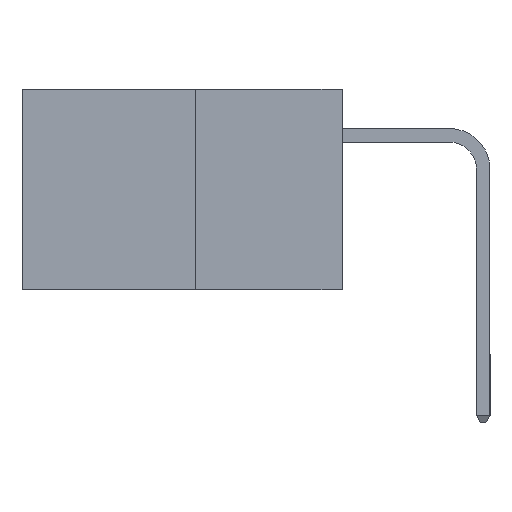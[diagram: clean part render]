
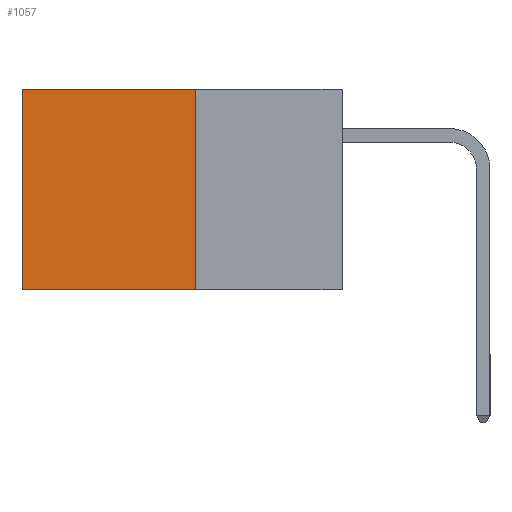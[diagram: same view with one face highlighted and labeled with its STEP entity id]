
A CAD part, left-side view. The second image highlights one B-rep face of the part: STEP entity #1057.
In plain terms, the highlighted planar face has unit normal (-1, 0, 0).
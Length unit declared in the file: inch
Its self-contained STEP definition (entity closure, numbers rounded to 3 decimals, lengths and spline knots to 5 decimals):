
#285 = EDGE_CURVE ( 'NONE', #2312, #536, #2381, .T. ) ;
#536 = VERTEX_POINT ( 'NONE', #2573 ) ;
#786 = AXIS2_PLACEMENT_3D ( 'NONE', #897, #1682, #1650 ) ;
#791 = EDGE_CURVE ( 'NONE', #8427, #2896, #4890, .T. ) ;
#897 = CARTESIAN_POINT ( 'NONE',  ( 0.277, 0.27, -0.37 ) ) ;
#1057 = ADVANCED_FACE ( 'NONE', ( #3097 ), #3990, .F. ) ;
#1630 = VECTOR ( 'NONE', #3398, 39.37008 ) ;
#1650 = DIRECTION ( 'NONE',  ( 0., 0., -1. ) ) ;
#1682 = DIRECTION ( 'NONE',  ( 1., 0., 0. ) ) ;
#2312 = VERTEX_POINT ( 'NONE', #4404 ) ;
#2381 = LINE ( 'NONE', #9972, #10028 ) ;
#2438 = CARTESIAN_POINT ( 'NONE',  ( 0.277, 0.27, -0.37 ) ) ;
#2573 = CARTESIAN_POINT ( 'NONE',  ( 0.277, 0.59, -0.37 ) ) ;
#2896 = VERTEX_POINT ( 'NONE', #2438 ) ;
#3097 = FACE_OUTER_BOUND ( 'NONE', #4039, .T. ) ;
#3225 = ORIENTED_EDGE ( 'NONE', *, *, #791, .F. ) ;
#3398 = DIRECTION ( 'NONE',  ( 0., 1., 0. ) ) ;
#3537 = CARTESIAN_POINT ( 'NONE',  ( 0.277, 0.27, 0. ) ) ;
#3704 = LINE ( 'NONE', #3537, #1630 ) ;
#3751 = EDGE_CURVE ( 'NONE', #8427, #2312, #3704, .T. ) ;
#3990 = PLANE ( 'NONE',  #786 ) ;
#4039 = EDGE_LOOP ( 'NONE', ( #5039, #7124, #3225, #5268 ) ) ;
#4404 = CARTESIAN_POINT ( 'NONE',  ( 0.277, 0.59, 0. ) ) ;
#4561 = DIRECTION ( 'NONE',  ( 0., 0., -1. ) ) ;
#4890 = LINE ( 'NONE', #6317, #8816 ) ;
#5039 = ORIENTED_EDGE ( 'NONE', *, *, #285, .T. ) ;
#5103 = CARTESIAN_POINT ( 'NONE',  ( 0.277, 0.27, 0. ) ) ;
#5268 = ORIENTED_EDGE ( 'NONE', *, *, #3751, .T. ) ;
#5277 = EDGE_CURVE ( 'NONE', #2896, #536, #5537, .T. ) ;
#5537 = LINE ( 'NONE', #7700, #7381 ) ;
#6317 = CARTESIAN_POINT ( 'NONE',  ( 0.277, 0.27, -0.37 ) ) ;
#7124 = ORIENTED_EDGE ( 'NONE', *, *, #5277, .F. ) ;
#7381 = VECTOR ( 'NONE', #7396, 39.37008 ) ;
#7396 = DIRECTION ( 'NONE',  ( 0., 1., 0. ) ) ;
#7700 = CARTESIAN_POINT ( 'NONE',  ( 0.277, 0.27, -0.37 ) ) ;
#8427 = VERTEX_POINT ( 'NONE', #5103 ) ;
#8816 = VECTOR ( 'NONE', #4561, 39.37008 ) ;
#9819 = DIRECTION ( 'NONE',  ( 0., 0., -1. ) ) ;
#9972 = CARTESIAN_POINT ( 'NONE',  ( 0.277, 0.59, -0.37 ) ) ;
#10028 = VECTOR ( 'NONE', #9819, 39.37008 ) ;
